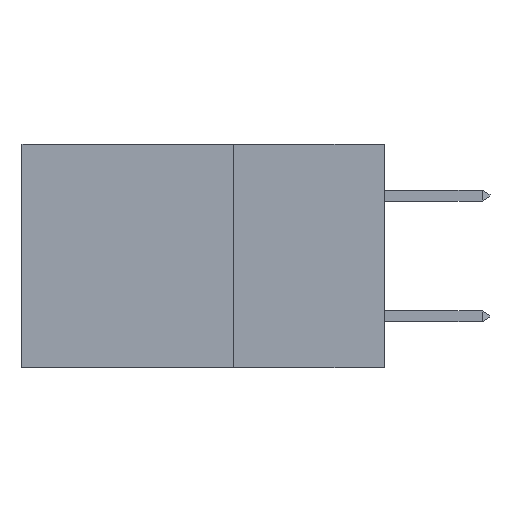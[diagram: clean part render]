
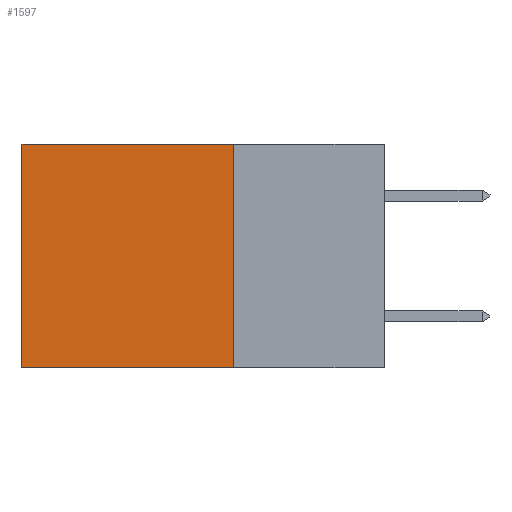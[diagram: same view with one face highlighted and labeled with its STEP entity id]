
A CAD part, left-side view. The second image highlights one B-rep face of the part: STEP entity #1597.
In plain terms, the highlighted planar face has unit normal (-1, 0, 0).
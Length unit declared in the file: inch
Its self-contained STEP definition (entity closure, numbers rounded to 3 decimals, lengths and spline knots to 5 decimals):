
#424 = EDGE_CURVE ( 'NONE', #1594, #1736, #13042, .T. ) ;
#497 = CARTESIAN_POINT ( 'NONE',  ( 0.2875, 0.25, 0. ) ) ;
#855 = CARTESIAN_POINT ( 'NONE',  ( 0.2875, 0.25, -0.37 ) ) ;
#933 = DIRECTION ( 'NONE',  ( 0., 1., 0. ) ) ;
#1238 = VECTOR ( 'NONE', #16129, 39.37008 ) ;
#1515 = VERTEX_POINT ( 'NONE', #5301 ) ;
#1594 = VERTEX_POINT ( 'NONE', #3718 ) ;
#1597 = ADVANCED_FACE ( 'NONE', ( #8434 ), #18477, .F. ) ;
#1736 = VERTEX_POINT ( 'NONE', #6456 ) ;
#1792 = EDGE_CURVE ( 'NONE', #4718, #1736, #11838, .T. ) ;
#3718 = CARTESIAN_POINT ( 'NONE',  ( 0.2875, 0.6, 0. ) ) ;
#3749 = VECTOR ( 'NONE', #933, 39.37008 ) ;
#3778 = ORIENTED_EDGE ( 'NONE', *, *, #1792, .F. ) ;
#3823 = LINE ( 'NONE', #19805, #1238 ) ;
#4718 = VERTEX_POINT ( 'NONE', #22600 ) ;
#5301 = CARTESIAN_POINT ( 'NONE',  ( 0.2875, 0.25, 0. ) ) ;
#6456 = CARTESIAN_POINT ( 'NONE',  ( 0.2875, 0.6, -0.37 ) ) ;
#8434 = FACE_OUTER_BOUND ( 'NONE', #23797, .T. ) ;
#9364 = AXIS2_PLACEMENT_3D ( 'NONE', #497, #11615, #19095 ) ;
#10280 = ORIENTED_EDGE ( 'NONE', *, *, #16010, .F. ) ;
#10494 = LINE ( 'NONE', #19063, #13264 ) ;
#11123 = ORIENTED_EDGE ( 'NONE', *, *, #424, .T. ) ;
#11615 = DIRECTION ( 'NONE',  ( 1., 0., 0. ) ) ;
#11838 = LINE ( 'NONE', #855, #3749 ) ;
#13042 = LINE ( 'NONE', #22346, #20542 ) ;
#13264 = VECTOR ( 'NONE', #20919, 39.37008 ) ;
#14950 = ORIENTED_EDGE ( 'NONE', *, *, #20193, .T. ) ;
#16010 = EDGE_CURVE ( 'NONE', #1515, #4718, #10494, .T. ) ;
#16129 = DIRECTION ( 'NONE',  ( 0., 1., 0. ) ) ;
#18477 = PLANE ( 'NONE',  #9364 ) ;
#18523 = DIRECTION ( 'NONE',  ( 0., 0., -1. ) ) ;
#19063 = CARTESIAN_POINT ( 'NONE',  ( 0.2875, 0.25, 0. ) ) ;
#19095 = DIRECTION ( 'NONE',  ( 0., 0., -1. ) ) ;
#19805 = CARTESIAN_POINT ( 'NONE',  ( 0.2875, 0.25, 0. ) ) ;
#20193 = EDGE_CURVE ( 'NONE', #1515, #1594, #3823, .T. ) ;
#20542 = VECTOR ( 'NONE', #18523, 39.37008 ) ;
#20919 = DIRECTION ( 'NONE',  ( 0., 0., -1. ) ) ;
#22346 = CARTESIAN_POINT ( 'NONE',  ( 0.2875, 0.6, 0. ) ) ;
#22600 = CARTESIAN_POINT ( 'NONE',  ( 0.2875, 0.25, -0.37 ) ) ;
#23797 = EDGE_LOOP ( 'NONE', ( #11123, #3778, #10280, #14950 ) ) ;
